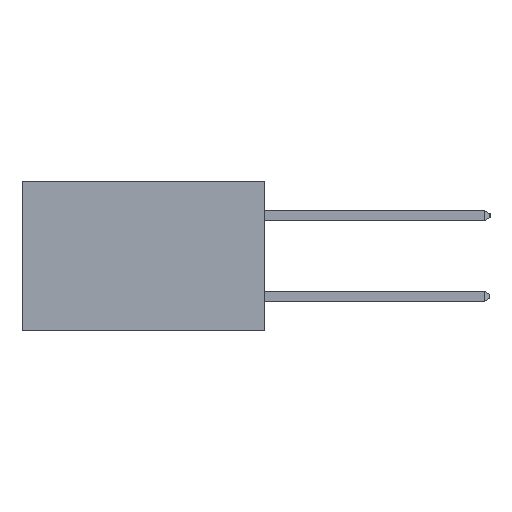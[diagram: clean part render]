
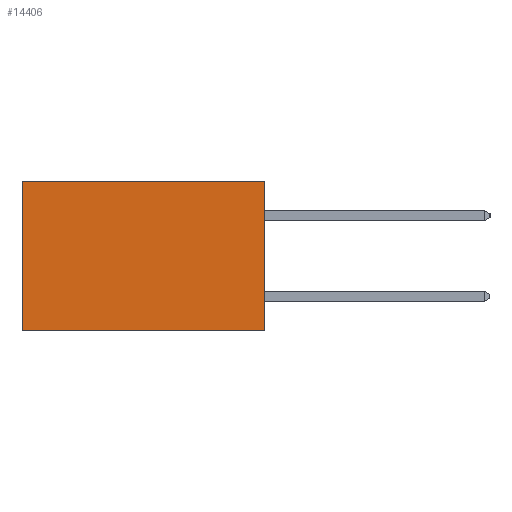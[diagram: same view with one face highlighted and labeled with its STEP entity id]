
A CAD part, left-side view. The second image highlights one B-rep face of the part: STEP entity #14406.
In plain terms, the highlighted planar face has unit normal (-1, 0, 0).
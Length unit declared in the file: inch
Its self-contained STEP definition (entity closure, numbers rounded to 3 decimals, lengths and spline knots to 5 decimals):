
#533 = VECTOR ( 'NONE', #12649, 39.37008 ) ;
#1013 = VERTEX_POINT ( 'NONE', #18181 ) ;
#2222 = CARTESIAN_POINT ( 'NONE',  ( 0.2615, 0.6, -0.37 ) ) ;
#4311 = LINE ( 'NONE', #10588, #8622 ) ;
#4447 = EDGE_CURVE ( 'NONE', #7036, #14715, #4311, .T. ) ;
#4587 = VERTEX_POINT ( 'NONE', #19330 ) ;
#5001 = EDGE_CURVE ( 'NONE', #1013, #4587, #11185, .T. ) ;
#6372 = EDGE_CURVE ( 'NONE', #4587, #14715, #12919, .T. ) ;
#7036 = VERTEX_POINT ( 'NONE', #9218 ) ;
#7180 = DIRECTION ( 'NONE',  ( 0., 0., -1. ) ) ;
#7358 = EDGE_LOOP ( 'NONE', ( #19971, #9406, #8076, #17116 ) ) ;
#8076 = ORIENTED_EDGE ( 'NONE', *, *, #5001, .F. ) ;
#8622 = VECTOR ( 'NONE', #14072, 39.37008 ) ;
#9218 = CARTESIAN_POINT ( 'NONE',  ( 0.2615, 0.6, 0. ) ) ;
#9394 = AXIS2_PLACEMENT_3D ( 'NONE', #19697, #18366, #7180 ) ;
#9406 = ORIENTED_EDGE ( 'NONE', *, *, #6372, .F. ) ;
#10529 = EDGE_CURVE ( 'NONE', #1013, #7036, #17330, .T. ) ;
#10588 = CARTESIAN_POINT ( 'NONE',  ( 0.2615, 0.6, -0.37 ) ) ;
#11185 = LINE ( 'NONE', #17390, #17726 ) ;
#11378 = DIRECTION ( 'NONE',  ( 0., 1., 0. ) ) ;
#12595 = VECTOR ( 'NONE', #11378, 39.37008 ) ;
#12649 = DIRECTION ( 'NONE',  ( 0., 1., 0. ) ) ;
#12919 = LINE ( 'NONE', #19116, #12595 ) ;
#14072 = DIRECTION ( 'NONE',  ( 0., 0., -1. ) ) ;
#14276 = CARTESIAN_POINT ( 'NONE',  ( 0.2615, 0., 0. ) ) ;
#14406 = ADVANCED_FACE ( 'NONE', ( #16951 ), #18271, .F. ) ;
#14715 = VERTEX_POINT ( 'NONE', #2222 ) ;
#15856 = DIRECTION ( 'NONE',  ( 0., 0., -1. ) ) ;
#16951 = FACE_OUTER_BOUND ( 'NONE', #7358, .T. ) ;
#17116 = ORIENTED_EDGE ( 'NONE', *, *, #10529, .T. ) ;
#17330 = LINE ( 'NONE', #14276, #533 ) ;
#17390 = CARTESIAN_POINT ( 'NONE',  ( 0.2615, 0., -0.37 ) ) ;
#17726 = VECTOR ( 'NONE', #15856, 39.37008 ) ;
#18181 = CARTESIAN_POINT ( 'NONE',  ( 0.2615, 0., 0. ) ) ;
#18271 = PLANE ( 'NONE',  #9394 ) ;
#18366 = DIRECTION ( 'NONE',  ( 1., 0., 0. ) ) ;
#19116 = CARTESIAN_POINT ( 'NONE',  ( 0.2615, 0., -0.37 ) ) ;
#19330 = CARTESIAN_POINT ( 'NONE',  ( 0.2615, 0., -0.37 ) ) ;
#19697 = CARTESIAN_POINT ( 'NONE',  ( 0.2615, 0., -0.37 ) ) ;
#19971 = ORIENTED_EDGE ( 'NONE', *, *, #4447, .T. ) ;
